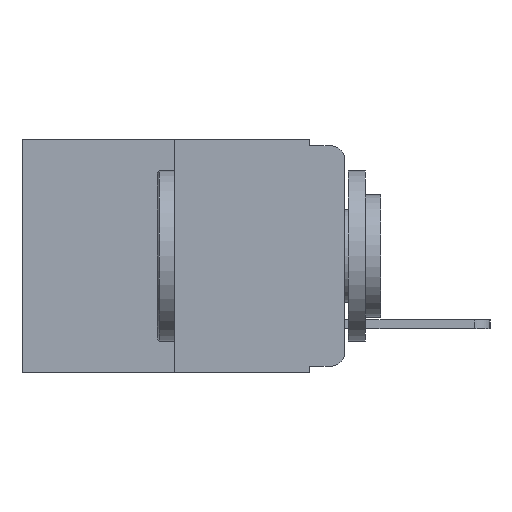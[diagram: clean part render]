
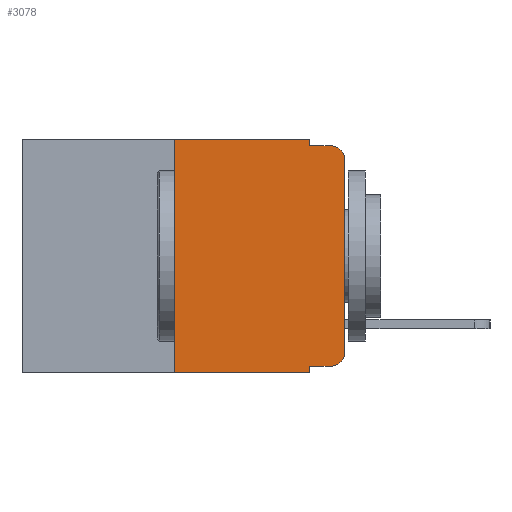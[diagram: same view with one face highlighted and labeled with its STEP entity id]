
A CAD part, left-side view. The second image highlights one B-rep face of the part: STEP entity #3078.
In plain terms, the highlighted planar face has unit normal (-1, 0, 0).
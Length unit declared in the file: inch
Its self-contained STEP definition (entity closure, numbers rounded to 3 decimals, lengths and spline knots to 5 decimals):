
#35 = CARTESIAN_POINT ( 'NONE',  ( 0., 0.473, -0.343 ) ) ;
#203 = ORIENTED_EDGE ( 'NONE', *, *, #5387, .T. ) ;
#349 = EDGE_CURVE ( 'NONE', #10356, #13726, #13183, .T. ) ;
#671 = PLANE ( 'NONE',  #10454 ) ;
#835 = VERTEX_POINT ( 'NONE', #12498 ) ;
#980 = EDGE_CURVE ( 'NONE', #2285, #5859, #11660, .T. ) ;
#1224 = ORIENTED_EDGE ( 'NONE', *, *, #349, .F. ) ;
#1482 = LINE ( 'NONE', #6533, #7939 ) ;
#1581 = ORIENTED_EDGE ( 'NONE', *, *, #7071, .F. ) ;
#1611 = AXIS2_PLACEMENT_3D ( 'NONE', #10415, #12764, #10362 ) ;
#1658 = CARTESIAN_POINT ( 'NONE',  ( 0., 0., -0.313 ) ) ;
#1771 = ORIENTED_EDGE ( 'NONE', *, *, #6813, .F. ) ;
#1806 = ORIENTED_EDGE ( 'NONE', *, *, #980, .T. ) ;
#1841 = ORIENTED_EDGE ( 'NONE', *, *, #14876, .T. ) ;
#1969 = ORIENTED_EDGE ( 'NONE', *, *, #8451, .F. ) ;
#2006 = ORIENTED_EDGE ( 'NONE', *, *, #6763, .F. ) ;
#2153 = CARTESIAN_POINT ( 'NONE',  ( 0., 0.051, -0.333 ) ) ;
#2285 = VERTEX_POINT ( 'NONE', #13322 ) ;
#2747 = LINE ( 'NONE', #12642, #15987 ) ;
#2945 = DIRECTION ( 'NONE',  ( 0., 0., -1. ) ) ;
#3078 = ADVANCED_FACE ( 'NONE', ( #7592 ), #671, .F. ) ;
#3215 = CARTESIAN_POINT ( 'NONE',  ( 0., 0.051, -0.01 ) ) ;
#3455 = CARTESIAN_POINT ( 'NONE',  ( 0., 0.02, -0.01 ) ) ;
#3790 = VECTOR ( 'NONE', #5314, 39.37008 ) ;
#4595 = LINE ( 'NONE', #14446, #14064 ) ;
#4625 = CARTESIAN_POINT ( 'NONE',  ( 0., 0.473, 0. ) ) ;
#4660 = DIRECTION ( 'NONE',  ( 0., -1., 0. ) ) ;
#4770 = LINE ( 'NONE', #35, #14610 ) ;
#4837 = CARTESIAN_POINT ( 'NONE',  ( 0., 0.051, -0.01 ) ) ;
#5207 = CARTESIAN_POINT ( 'NONE',  ( 0., 0.25, 0. ) ) ;
#5314 = DIRECTION ( 'NONE',  ( 0., -1., 0. ) ) ;
#5387 = EDGE_CURVE ( 'NONE', #835, #2285, #15186, .T. ) ;
#5725 = VECTOR ( 'NONE', #11911, 39.37008 ) ;
#5859 = VERTEX_POINT ( 'NONE', #1658 ) ;
#6361 = DIRECTION ( 'NONE',  ( 0., 0., -1. ) ) ;
#6440 = DIRECTION ( 'NONE',  ( -1., 0., 0. ) ) ;
#6454 = EDGE_CURVE ( 'NONE', #9365, #13726, #13191, .T. ) ;
#6533 = CARTESIAN_POINT ( 'NONE',  ( 0., 0., 0. ) ) ;
#6654 = CARTESIAN_POINT ( 'NONE',  ( 0., 0.25, -0.343 ) ) ;
#6763 = EDGE_CURVE ( 'NONE', #13366, #8436, #4595, .T. ) ;
#6813 = EDGE_CURVE ( 'NONE', #8436, #8127, #10441, .T. ) ;
#7071 = EDGE_CURVE ( 'NONE', #835, #11114, #11956, .T. ) ;
#7592 = FACE_OUTER_BOUND ( 'NONE', #12691, .T. ) ;
#7939 = VECTOR ( 'NONE', #11084, 39.37008 ) ;
#8127 = VERTEX_POINT ( 'NONE', #8999 ) ;
#8134 = EDGE_CURVE ( 'NONE', #5859, #9365, #1482, .T. ) ;
#8436 = VERTEX_POINT ( 'NONE', #5207 ) ;
#8451 = EDGE_CURVE ( 'NONE', #8127, #10356, #2747, .T. ) ;
#8936 = ORIENTED_EDGE ( 'NONE', *, *, #8134, .T. ) ;
#8999 = CARTESIAN_POINT ( 'NONE',  ( 0., 0.051, 0. ) ) ;
#9045 = DIRECTION ( 'NONE',  ( 0., -1., 0. ) ) ;
#9210 = VECTOR ( 'NONE', #4660, 39.37008 ) ;
#9365 = VERTEX_POINT ( 'NONE', #10757 ) ;
#9603 = DIRECTION ( 'NONE',  ( 0., 0., 1. ) ) ;
#9688 = DIRECTION ( 'NONE',  ( 0., 0., -1. ) ) ;
#10356 = VERTEX_POINT ( 'NONE', #3215 ) ;
#10362 = DIRECTION ( 'NONE',  ( 0., 0., -1. ) ) ;
#10415 = CARTESIAN_POINT ( 'NONE',  ( 0., 0.02, -0.313 ) ) ;
#10441 = LINE ( 'NONE', #11263, #3790 ) ;
#10454 = AXIS2_PLACEMENT_3D ( 'NONE', #4625, #11526, #2945 ) ;
#10757 = CARTESIAN_POINT ( 'NONE',  ( 0., 0., -0.03 ) ) ;
#11084 = DIRECTION ( 'NONE',  ( 0., 0., 1. ) ) ;
#11114 = VERTEX_POINT ( 'NONE', #13508 ) ;
#11263 = CARTESIAN_POINT ( 'NONE',  ( 0., 0.473, 0. ) ) ;
#11421 = DIRECTION ( 'NONE',  ( 0., 0., -1. ) ) ;
#11512 = CARTESIAN_POINT ( 'NONE',  ( 0., 0.02, -0.03 ) ) ;
#11526 = DIRECTION ( 'NONE',  ( 1., 0., 0. ) ) ;
#11572 = ORIENTED_EDGE ( 'NONE', *, *, #6454, .T. ) ;
#11660 = CIRCLE ( 'NONE', #1611, 0.02 ) ;
#11911 = DIRECTION ( 'NONE',  ( 0., -1., 0. ) ) ;
#11956 = LINE ( 'NONE', #16088, #14828 ) ;
#12498 = CARTESIAN_POINT ( 'NONE',  ( 0., 0.051, -0.333 ) ) ;
#12642 = CARTESIAN_POINT ( 'NONE',  ( 0., 0.051, 0. ) ) ;
#12691 = EDGE_LOOP ( 'NONE', ( #8936, #11572, #1224, #1969, #1771, #2006, #1841, #1581, #203, #1806 ) ) ;
#12764 = DIRECTION ( 'NONE',  ( -1., 0., 0. ) ) ;
#13183 = LINE ( 'NONE', #4837, #9210 ) ;
#13191 = CIRCLE ( 'NONE', #15633, 0.02 ) ;
#13322 = CARTESIAN_POINT ( 'NONE',  ( 0., 0.02, -0.333 ) ) ;
#13366 = VERTEX_POINT ( 'NONE', #6654 ) ;
#13508 = CARTESIAN_POINT ( 'NONE',  ( 0., 0.051, -0.343 ) ) ;
#13726 = VERTEX_POINT ( 'NONE', #3455 ) ;
#14064 = VECTOR ( 'NONE', #9603, 39.37008 ) ;
#14446 = CARTESIAN_POINT ( 'NONE',  ( 0., 0.25, 0. ) ) ;
#14610 = VECTOR ( 'NONE', #9045, 39.37008 ) ;
#14828 = VECTOR ( 'NONE', #9688, 39.37008 ) ;
#14876 = EDGE_CURVE ( 'NONE', #13366, #11114, #4770, .T. ) ;
#15186 = LINE ( 'NONE', #2153, #5725 ) ;
#15633 = AXIS2_PLACEMENT_3D ( 'NONE', #11512, #6440, #6361 ) ;
#15987 = VECTOR ( 'NONE', #11421, 39.37008 ) ;
#16088 = CARTESIAN_POINT ( 'NONE',  ( 0., 0.051, 0. ) ) ;
